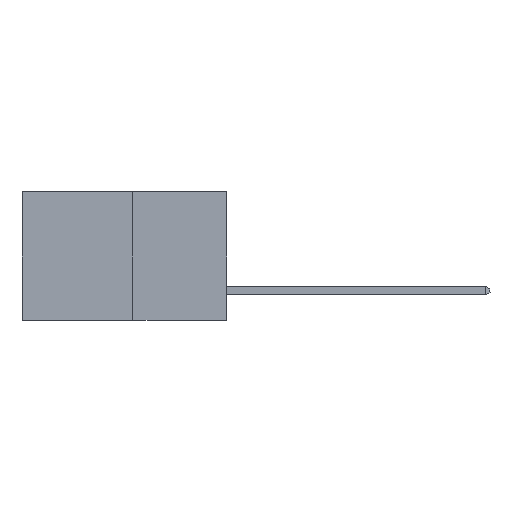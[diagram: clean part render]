
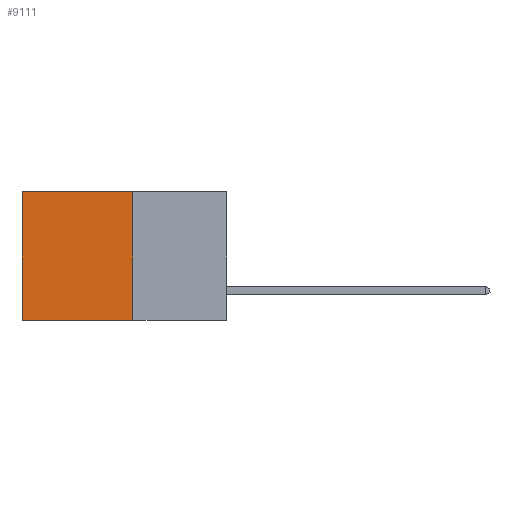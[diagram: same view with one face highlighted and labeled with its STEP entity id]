
A CAD part, left-side view. The second image highlights one B-rep face of the part: STEP entity #9111.
In plain terms, the highlighted planar face has unit normal (-1, 0, 0).
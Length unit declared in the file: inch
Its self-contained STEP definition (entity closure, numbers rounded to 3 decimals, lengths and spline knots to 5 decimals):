
#368 = DIRECTION ( 'NONE',  ( 0., 1., 0. ) ) ;
#471 = CARTESIAN_POINT ( 'NONE',  ( 0.277, 0.27, -0.37 ) ) ;
#967 = VERTEX_POINT ( 'NONE', #8838 ) ;
#1470 = VERTEX_POINT ( 'NONE', #3743 ) ;
#1753 = VERTEX_POINT ( 'NONE', #3266 ) ;
#1984 = EDGE_CURVE ( 'NONE', #967, #1470, #8574, .T. ) ;
#2468 = AXIS2_PLACEMENT_3D ( 'NONE', #8946, #9755, #4638 ) ;
#2928 = PLANE ( 'NONE',  #2468 ) ;
#3266 = CARTESIAN_POINT ( 'NONE',  ( 0.277, 0.27, 0. ) ) ;
#3377 = EDGE_LOOP ( 'NONE', ( #7241, #7770, #6565, #4774 ) ) ;
#3709 = EDGE_CURVE ( 'NONE', #9234, #1470, #9441, .T. ) ;
#3743 = CARTESIAN_POINT ( 'NONE',  ( 0.277, 0.59, -0.37 ) ) ;
#3800 = CARTESIAN_POINT ( 'NONE',  ( 0.277, 0.27, -0.37 ) ) ;
#3904 = CARTESIAN_POINT ( 'NONE',  ( 0.277, 0.27, 0. ) ) ;
#4638 = DIRECTION ( 'NONE',  ( 0., 0., -1. ) ) ;
#4774 = ORIENTED_EDGE ( 'NONE', *, *, #8617, .T. ) ;
#4887 = VECTOR ( 'NONE', #368, 39.37008 ) ;
#5541 = LINE ( 'NONE', #3904, #7853 ) ;
#5680 = CARTESIAN_POINT ( 'NONE',  ( 0.277, 0.27, -0.37 ) ) ;
#6291 = VECTOR ( 'NONE', #10830, 39.37008 ) ;
#6371 = LINE ( 'NONE', #3800, #8392 ) ;
#6565 = ORIENTED_EDGE ( 'NONE', *, *, #8532, .F. ) ;
#7241 = ORIENTED_EDGE ( 'NONE', *, *, #1984, .T. ) ;
#7770 = ORIENTED_EDGE ( 'NONE', *, *, #3709, .F. ) ;
#7853 = VECTOR ( 'NONE', #9875, 39.37008 ) ;
#8392 = VECTOR ( 'NONE', #10548, 39.37008 ) ;
#8532 = EDGE_CURVE ( 'NONE', #1753, #9234, #6371, .T. ) ;
#8574 = LINE ( 'NONE', #10947, #6291 ) ;
#8617 = EDGE_CURVE ( 'NONE', #1753, #967, #5541, .T. ) ;
#8757 = FACE_OUTER_BOUND ( 'NONE', #3377, .T. ) ;
#8838 = CARTESIAN_POINT ( 'NONE',  ( 0.277, 0.59, 0. ) ) ;
#8946 = CARTESIAN_POINT ( 'NONE',  ( 0.277, 0.27, -0.37 ) ) ;
#9111 = ADVANCED_FACE ( 'NONE', ( #8757 ), #2928, .F. ) ;
#9234 = VERTEX_POINT ( 'NONE', #5680 ) ;
#9441 = LINE ( 'NONE', #471, #4887 ) ;
#9755 = DIRECTION ( 'NONE',  ( 1., 0., 0. ) ) ;
#9875 = DIRECTION ( 'NONE',  ( 0., 1., 0. ) ) ;
#10548 = DIRECTION ( 'NONE',  ( 0., 0., -1. ) ) ;
#10830 = DIRECTION ( 'NONE',  ( 0., 0., -1. ) ) ;
#10947 = CARTESIAN_POINT ( 'NONE',  ( 0.277, 0.59, -0.37 ) ) ;
